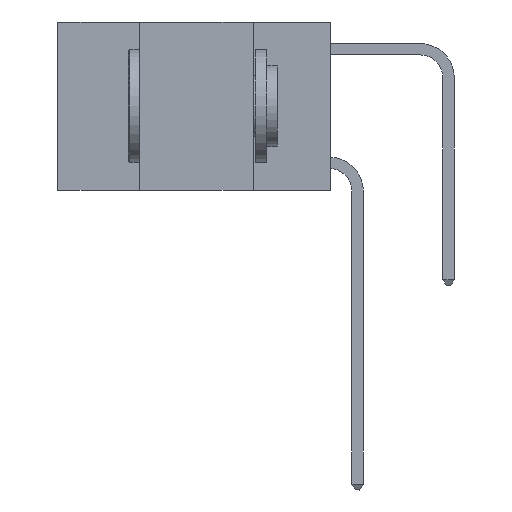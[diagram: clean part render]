
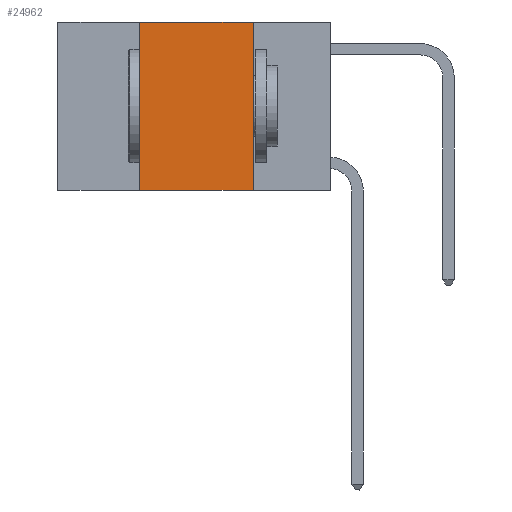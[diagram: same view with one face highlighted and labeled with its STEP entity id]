
A CAD part, left-side view. The second image highlights one B-rep face of the part: STEP entity #24962.
In plain terms, the highlighted planar face has unit normal (-1, 0, 0).
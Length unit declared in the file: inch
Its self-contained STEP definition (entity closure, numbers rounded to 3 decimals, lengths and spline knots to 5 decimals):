
#1388 = LINE ( 'NONE', #20757, #20401 ) ;
#2131 = LINE ( 'NONE', #31227, #13795 ) ;
#3701 = ORIENTED_EDGE ( 'NONE', *, *, #7815, .T. ) ;
#4334 = VERTEX_POINT ( 'NONE', #20408 ) ;
#5354 = CARTESIAN_POINT ( 'NONE',  ( 0., 0.6, 0. ) ) ;
#5655 = VECTOR ( 'NONE', #28455, 39.37008 ) ;
#6463 = DIRECTION ( 'NONE',  ( 0., 0., 1. ) ) ;
#6581 = VECTOR ( 'NONE', #6463, 39.37008 ) ;
#7815 = EDGE_CURVE ( 'NONE', #11802, #8943, #13016, .T. ) ;
#7859 = DIRECTION ( 'NONE',  ( 0., 0., -1. ) ) ;
#7999 = ORIENTED_EDGE ( 'NONE', *, *, #19968, .F. ) ;
#8943 = VERTEX_POINT ( 'NONE', #20865 ) ;
#10620 = EDGE_LOOP ( 'NONE', ( #7999, #27739, #22700, #3701 ) ) ;
#11174 = FACE_OUTER_BOUND ( 'NONE', #10620, .T. ) ;
#11802 = VERTEX_POINT ( 'NONE', #21905 ) ;
#13016 = LINE ( 'NONE', #25941, #5655 ) ;
#13154 = LINE ( 'NONE', #30997, #6581 ) ;
#13795 = VECTOR ( 'NONE', #23791, 39.37008 ) ;
#16124 = EDGE_CURVE ( 'NONE', #11802, #4334, #13154, .T. ) ;
#17399 = EDGE_CURVE ( 'NONE', #4334, #19174, #1388, .T. ) ;
#19174 = VERTEX_POINT ( 'NONE', #30848 ) ;
#19968 = EDGE_CURVE ( 'NONE', #19174, #8943, #2131, .T. ) ;
#20401 = VECTOR ( 'NONE', #23257, 39.37008 ) ;
#20408 = CARTESIAN_POINT ( 'NONE',  ( 0., 0.42, 0. ) ) ;
#20757 = CARTESIAN_POINT ( 'NONE',  ( 0., 0.6, 0. ) ) ;
#20865 = CARTESIAN_POINT ( 'NONE',  ( 0., 0.17, -0.37 ) ) ;
#21905 = CARTESIAN_POINT ( 'NONE',  ( 0., 0.42, -0.37 ) ) ;
#22660 = DIRECTION ( 'NONE',  ( 1., 0., 0. ) ) ;
#22700 = ORIENTED_EDGE ( 'NONE', *, *, #16124, .F. ) ;
#23257 = DIRECTION ( 'NONE',  ( 0., -1., 0. ) ) ;
#23791 = DIRECTION ( 'NONE',  ( 0., 0., -1. ) ) ;
#24962 = ADVANCED_FACE ( 'NONE', ( #11174 ), #27543, .F. ) ;
#25941 = CARTESIAN_POINT ( 'NONE',  ( 0., 0.6, -0.37 ) ) ;
#26194 = AXIS2_PLACEMENT_3D ( 'NONE', #5354, #22660, #7859 ) ;
#27543 = PLANE ( 'NONE',  #26194 ) ;
#27739 = ORIENTED_EDGE ( 'NONE', *, *, #17399, .F. ) ;
#28455 = DIRECTION ( 'NONE',  ( 0., -1., 0. ) ) ;
#30848 = CARTESIAN_POINT ( 'NONE',  ( 0., 0.17, 0. ) ) ;
#30997 = CARTESIAN_POINT ( 'NONE',  ( 0., 0.42, 0. ) ) ;
#31227 = CARTESIAN_POINT ( 'NONE',  ( 0., 0.17, 0. ) ) ;
